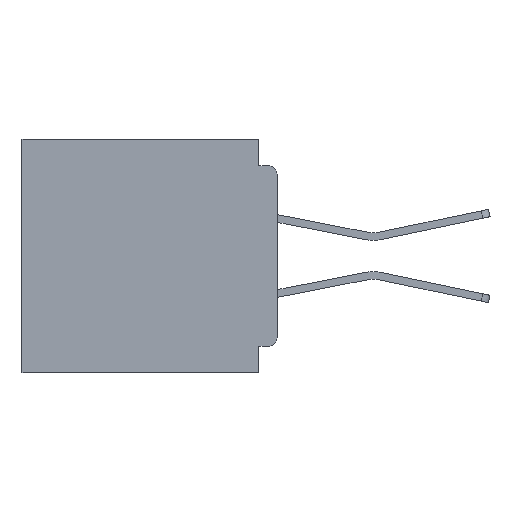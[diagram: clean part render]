
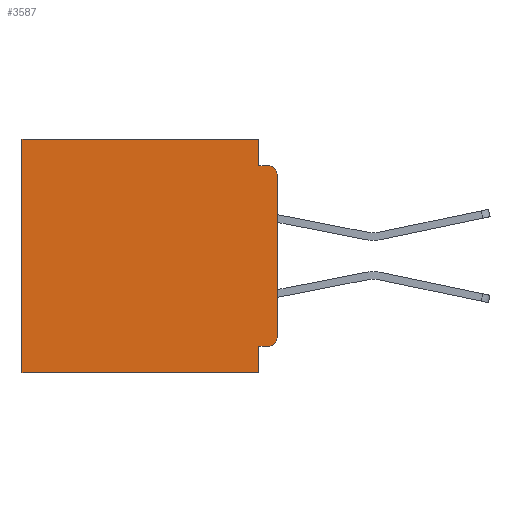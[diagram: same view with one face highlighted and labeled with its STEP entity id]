
A CAD part, left-side view. The second image highlights one B-rep face of the part: STEP entity #3587.
In plain terms, the highlighted planar face has unit normal (-1, 0, 0).
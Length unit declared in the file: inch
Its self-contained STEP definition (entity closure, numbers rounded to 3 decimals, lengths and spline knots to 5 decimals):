
#413 = CARTESIAN_POINT ( 'NONE',  ( 0.3, 0.031, 0. ) ) ;
#458 = ORIENTED_EDGE ( 'NONE', *, *, #43127, .F. ) ;
#462 = DIRECTION ( 'NONE',  ( 0., 0., -1. ) ) ;
#1397 = CARTESIAN_POINT ( 'NONE',  ( 0.3, 0., -0.34 ) ) ;
#1404 = VECTOR ( 'NONE', #3017, 39.37008 ) ;
#1553 = CARTESIAN_POINT ( 'NONE',  ( 0.3, 0., 0. ) ) ;
#2061 = CARTESIAN_POINT ( 'NONE',  ( 0.3, 0.031, -0.045 ) ) ;
#2106 = CARTESIAN_POINT ( 'NONE',  ( 0.3, 0.015, -0.34 ) ) ;
#2344 = EDGE_CURVE ( 'NONE', #41985, #43126, #12776, .T. ) ;
#2433 = VERTEX_POINT ( 'NONE', #41387 ) ;
#2541 = EDGE_CURVE ( 'NONE', #28148, #46339, #4489, .T. ) ;
#2628 = CARTESIAN_POINT ( 'NONE',  ( 0.3, 0.437, 0. ) ) ;
#3017 = DIRECTION ( 'NONE',  ( 0., 1., 0. ) ) ;
#3587 = ADVANCED_FACE ( 'NONE', ( #16186 ), #43917, .F. ) ;
#4176 = EDGE_CURVE ( 'NONE', #46690, #2433, #38557, .T. ) ;
#4489 = LINE ( 'NONE', #41869, #43289 ) ;
#4665 = CARTESIAN_POINT ( 'NONE',  ( 0.3, 0.031, -0.4 ) ) ;
#5326 = VERTEX_POINT ( 'NONE', #1397 ) ;
#5889 = DIRECTION ( 'NONE',  ( 0., 0., -1. ) ) ;
#6067 = CIRCLE ( 'NONE', #20964, 0.015 ) ;
#6402 = ORIENTED_EDGE ( 'NONE', *, *, #4176, .F. ) ;
#6552 = DIRECTION ( 'NONE',  ( 0., 0., -1. ) ) ;
#6685 = CARTESIAN_POINT ( 'NONE',  ( 0.3, 0.015, -0.355 ) ) ;
#7680 = VERTEX_POINT ( 'NONE', #6685 ) ;
#8135 = VECTOR ( 'NONE', #38573, 39.37008 ) ;
#9344 = LINE ( 'NONE', #4665, #8135 ) ;
#9352 = ORIENTED_EDGE ( 'NONE', *, *, #2541, .F. ) ;
#9949 = CARTESIAN_POINT ( 'NONE',  ( 0.3, 0., -0.06 ) ) ;
#10364 = CARTESIAN_POINT ( 'NONE',  ( 0.3, 0.031, 0. ) ) ;
#12017 = DIRECTION ( 'NONE',  ( 0., 1., 0. ) ) ;
#12124 = CARTESIAN_POINT ( 'NONE',  ( 0.3, 0.437, -0.4 ) ) ;
#12776 = LINE ( 'NONE', #1553, #31696 ) ;
#12835 = EDGE_LOOP ( 'NONE', ( #30307, #39352, #6402, #458, #48164, #17082, #9352, #16355, #40265, #48322 ) ) ;
#13894 = EDGE_CURVE ( 'NONE', #43126, #46339, #33784, .T. ) ;
#15430 = CARTESIAN_POINT ( 'NONE',  ( 0.3, 0., -0.4 ) ) ;
#15479 = VECTOR ( 'NONE', #6552, 39.37008 ) ;
#15918 = CARTESIAN_POINT ( 'NONE',  ( 0.3, 0.031, -0.4 ) ) ;
#16186 = FACE_OUTER_BOUND ( 'NONE', #12835, .T. ) ;
#16262 = CARTESIAN_POINT ( 'NONE',  ( 0.3, 0., -0.045 ) ) ;
#16355 = ORIENTED_EDGE ( 'NONE', *, *, #30651, .F. ) ;
#16689 = LINE ( 'NONE', #10364, #15479 ) ;
#17082 = ORIENTED_EDGE ( 'NONE', *, *, #13894, .T. ) ;
#18366 = DIRECTION ( 'NONE',  ( -1., 0., 0. ) ) ;
#18536 = DIRECTION ( 'NONE',  ( 0., 0., -1. ) ) ;
#18712 = EDGE_CURVE ( 'NONE', #23759, #2433, #6067, .T. ) ;
#18716 = DIRECTION ( 'NONE',  ( 1., 0., 0. ) ) ;
#19444 = AXIS2_PLACEMENT_3D ( 'NONE', #15430, #18716, #18536 ) ;
#19676 = AXIS2_PLACEMENT_3D ( 'NONE', #2106, #28519, #5889 ) ;
#20964 = AXIS2_PLACEMENT_3D ( 'NONE', #40851, #18366, #44535 ) ;
#23759 = VERTEX_POINT ( 'NONE', #9949 ) ;
#23803 = VECTOR ( 'NONE', #45868, 39.37008 ) ;
#28148 = VERTEX_POINT ( 'NONE', #15918 ) ;
#28325 = LINE ( 'NONE', #45266, #38239 ) ;
#28519 = DIRECTION ( 'NONE',  ( -1., 0., 0. ) ) ;
#29425 = CARTESIAN_POINT ( 'NONE',  ( 0.3, 0., -0.355 ) ) ;
#30307 = ORIENTED_EDGE ( 'NONE', *, *, #39500, .F. ) ;
#30651 = EDGE_CURVE ( 'NONE', #40946, #28148, #9344, .T. ) ;
#31696 = VECTOR ( 'NONE', #38733, 39.37008 ) ;
#33784 = LINE ( 'NONE', #12124, #23803 ) ;
#35335 = CIRCLE ( 'NONE', #19676, 0.015 ) ;
#35801 = CARTESIAN_POINT ( 'NONE',  ( 0.3, 0.031, -0.355 ) ) ;
#36385 = EDGE_CURVE ( 'NONE', #7680, #40946, #41398, .T. ) ;
#38239 = VECTOR ( 'NONE', #462, 39.37008 ) ;
#38557 = LINE ( 'NONE', #16262, #47216 ) ;
#38573 = DIRECTION ( 'NONE',  ( 0., 0., -1. ) ) ;
#38614 = DIRECTION ( 'NONE',  ( 0., -1., 0. ) ) ;
#38733 = DIRECTION ( 'NONE',  ( 0., 1., 0. ) ) ;
#39352 = ORIENTED_EDGE ( 'NONE', *, *, #18712, .T. ) ;
#39500 = EDGE_CURVE ( 'NONE', #23759, #5326, #28325, .T. ) ;
#39777 = EDGE_CURVE ( 'NONE', #7680, #5326, #35335, .T. ) ;
#40265 = ORIENTED_EDGE ( 'NONE', *, *, #36385, .F. ) ;
#40851 = CARTESIAN_POINT ( 'NONE',  ( 0.3, 0.015, -0.06 ) ) ;
#40946 = VERTEX_POINT ( 'NONE', #35801 ) ;
#41363 = CARTESIAN_POINT ( 'NONE',  ( 0.3, 0.437, -0.4 ) ) ;
#41387 = CARTESIAN_POINT ( 'NONE',  ( 0.3, 0.015, -0.045 ) ) ;
#41398 = LINE ( 'NONE', #29425, #1404 ) ;
#41869 = CARTESIAN_POINT ( 'NONE',  ( 0.3, 0., -0.4 ) ) ;
#41985 = VERTEX_POINT ( 'NONE', #413 ) ;
#43126 = VERTEX_POINT ( 'NONE', #2628 ) ;
#43127 = EDGE_CURVE ( 'NONE', #41985, #46690, #16689, .T. ) ;
#43289 = VECTOR ( 'NONE', #12017, 39.37008 ) ;
#43917 = PLANE ( 'NONE',  #19444 ) ;
#44535 = DIRECTION ( 'NONE',  ( 0., 0., -1. ) ) ;
#45266 = CARTESIAN_POINT ( 'NONE',  ( 0.3, 0., -0.4 ) ) ;
#45868 = DIRECTION ( 'NONE',  ( 0., 0., -1. ) ) ;
#46339 = VERTEX_POINT ( 'NONE', #41363 ) ;
#46690 = VERTEX_POINT ( 'NONE', #2061 ) ;
#47216 = VECTOR ( 'NONE', #38614, 39.37008 ) ;
#48164 = ORIENTED_EDGE ( 'NONE', *, *, #2344, .T. ) ;
#48322 = ORIENTED_EDGE ( 'NONE', *, *, #39777, .T. ) ;
